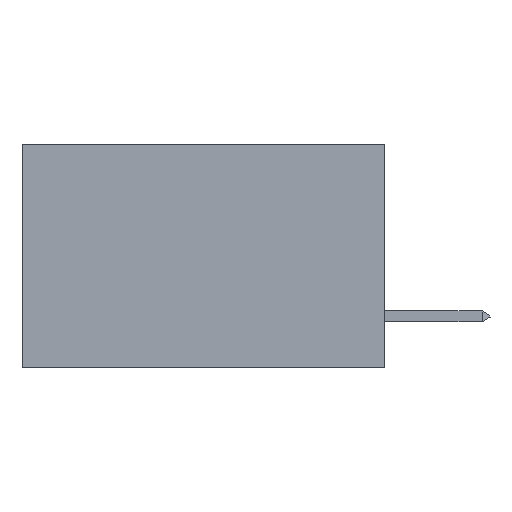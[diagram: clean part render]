
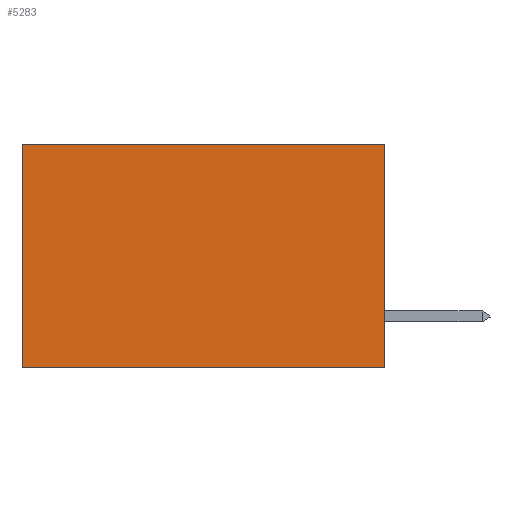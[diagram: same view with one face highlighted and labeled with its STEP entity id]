
A CAD part, left-side view. The second image highlights one B-rep face of the part: STEP entity #5283.
In plain terms, the highlighted planar face has unit normal (-1, 0, 0).
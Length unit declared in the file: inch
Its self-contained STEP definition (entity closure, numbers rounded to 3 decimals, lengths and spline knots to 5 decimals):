
#742 = VERTEX_POINT ( 'NONE', #17907 ) ;
#1222 = VECTOR ( 'NONE', #20320, 39.37008 ) ;
#1768 = VERTEX_POINT ( 'NONE', #21021 ) ;
#2999 = CARTESIAN_POINT ( 'NONE',  ( 0.2875, 0.6, -0.37 ) ) ;
#3198 = FACE_OUTER_BOUND ( 'NONE', #25684, .T. ) ;
#3904 = DIRECTION ( 'NONE',  ( 0., 0., -1. ) ) ;
#4422 = LINE ( 'NONE', #13405, #10493 ) ;
#4766 = ORIENTED_EDGE ( 'NONE', *, *, #7568, .T. ) ;
#5283 = ADVANCED_FACE ( 'NONE', ( #3198 ), #29138, .F. ) ;
#6782 = EDGE_CURVE ( 'NONE', #1768, #14725, #22698, .T. ) ;
#7568 = EDGE_CURVE ( 'NONE', #742, #14725, #4422, .T. ) ;
#7599 = EDGE_CURVE ( 'NONE', #27964, #742, #29441, .T. ) ;
#8034 = EDGE_CURVE ( 'NONE', #27964, #1768, #8278, .T. ) ;
#8278 = LINE ( 'NONE', #13173, #23680 ) ;
#8475 = ORIENTED_EDGE ( 'NONE', *, *, #6782, .F. ) ;
#9828 = VECTOR ( 'NONE', #24894, 39.37008 ) ;
#10493 = VECTOR ( 'NONE', #20124, 39.37008 ) ;
#12943 = CARTESIAN_POINT ( 'NONE',  ( 0.2875, 0., 0. ) ) ;
#13173 = CARTESIAN_POINT ( 'NONE',  ( 0.2875, 0., 0. ) ) ;
#13405 = CARTESIAN_POINT ( 'NONE',  ( 0.2875, 0.6, 0. ) ) ;
#14725 = VERTEX_POINT ( 'NONE', #2999 ) ;
#17893 = CARTESIAN_POINT ( 'NONE',  ( 0.2875, 0., -0.37 ) ) ;
#17907 = CARTESIAN_POINT ( 'NONE',  ( 0.2875, 0.6, 0. ) ) ;
#20124 = DIRECTION ( 'NONE',  ( 0., 0., -1. ) ) ;
#20320 = DIRECTION ( 'NONE',  ( 0., 1., 0. ) ) ;
#20921 = ORIENTED_EDGE ( 'NONE', *, *, #8034, .F. ) ;
#21021 = CARTESIAN_POINT ( 'NONE',  ( 0.2875, 0., -0.37 ) ) ;
#21578 = AXIS2_PLACEMENT_3D ( 'NONE', #12943, #27015, #3904 ) ;
#22698 = LINE ( 'NONE', #17893, #9828 ) ;
#23680 = VECTOR ( 'NONE', #29263, 39.37008 ) ;
#24795 = CARTESIAN_POINT ( 'NONE',  ( 0.2875, 0., 0. ) ) ;
#24894 = DIRECTION ( 'NONE',  ( 0., 1., 0. ) ) ;
#25379 = ORIENTED_EDGE ( 'NONE', *, *, #7599, .T. ) ;
#25684 = EDGE_LOOP ( 'NONE', ( #4766, #8475, #20921, #25379 ) ) ;
#26191 = CARTESIAN_POINT ( 'NONE',  ( 0.2875, 0., 0. ) ) ;
#27015 = DIRECTION ( 'NONE',  ( 1., 0., 0. ) ) ;
#27964 = VERTEX_POINT ( 'NONE', #26191 ) ;
#29138 = PLANE ( 'NONE',  #21578 ) ;
#29263 = DIRECTION ( 'NONE',  ( 0., 0., -1. ) ) ;
#29441 = LINE ( 'NONE', #24795, #1222 ) ;
